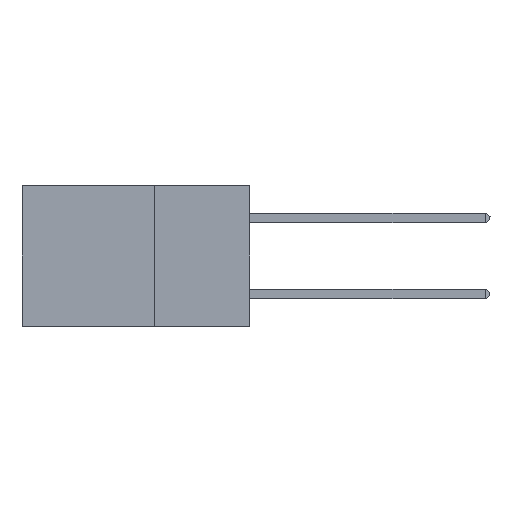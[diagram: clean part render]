
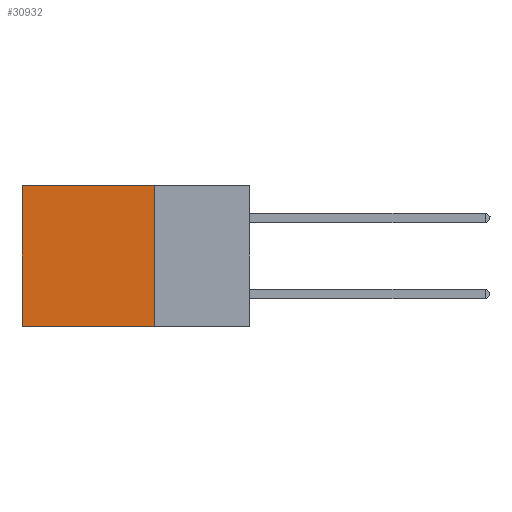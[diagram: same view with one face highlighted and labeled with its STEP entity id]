
A CAD part, left-side view. The second image highlights one B-rep face of the part: STEP entity #30932.
In plain terms, the highlighted planar face has unit normal (-1, 0, 0).
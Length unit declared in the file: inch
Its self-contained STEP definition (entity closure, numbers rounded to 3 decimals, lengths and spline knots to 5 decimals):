
#968 = VERTEX_POINT ( 'NONE', #5700 ) ;
#1613 = VERTEX_POINT ( 'NONE', #4851 ) ;
#2082 = ORIENTED_EDGE ( 'NONE', *, *, #34504, .F. ) ;
#3771 = LINE ( 'NONE', #9595, #23600 ) ;
#3951 = DIRECTION ( 'NONE',  ( 0., 0., -1. ) ) ;
#4851 = CARTESIAN_POINT ( 'NONE',  ( 0.2875, 0.6, -0.37 ) ) ;
#4903 = PLANE ( 'NONE',  #20054 ) ;
#5700 = CARTESIAN_POINT ( 'NONE',  ( 0.2875, 0.6, 0. ) ) ;
#8039 = CARTESIAN_POINT ( 'NONE',  ( 0.2875, 0.25, -0.37 ) ) ;
#9595 = CARTESIAN_POINT ( 'NONE',  ( 0.2875, 0.6, 0. ) ) ;
#10537 = FACE_OUTER_BOUND ( 'NONE', #33768, .T. ) ;
#10562 = EDGE_CURVE ( 'NONE', #968, #1613, #3771, .T. ) ;
#10902 = CARTESIAN_POINT ( 'NONE',  ( 0.2875, 0.25, 0. ) ) ;
#11236 = ORIENTED_EDGE ( 'NONE', *, *, #29408, .T. ) ;
#11435 = VECTOR ( 'NONE', #25036, 39.37008 ) ;
#13831 = DIRECTION ( 'NONE',  ( 1., 0., 0. ) ) ;
#14778 = ORIENTED_EDGE ( 'NONE', *, *, #35488, .F. ) ;
#17327 = VERTEX_POINT ( 'NONE', #25111 ) ;
#19343 = CARTESIAN_POINT ( 'NONE',  ( 0.2875, 0.25, 0. ) ) ;
#20054 = AXIS2_PLACEMENT_3D ( 'NONE', #10902, #13831, #33153 ) ;
#21034 = CARTESIAN_POINT ( 'NONE',  ( 0.2875, 0.25, -0.37 ) ) ;
#23600 = VECTOR ( 'NONE', #3951, 39.37008 ) ;
#23776 = LINE ( 'NONE', #21034, #24204 ) ;
#24204 = VECTOR ( 'NONE', #27042, 39.37008 ) ;
#24647 = VERTEX_POINT ( 'NONE', #8039 ) ;
#25036 = DIRECTION ( 'NONE',  ( 0., 0., -1. ) ) ;
#25111 = CARTESIAN_POINT ( 'NONE',  ( 0.2875, 0.25, 0. ) ) ;
#25226 = CARTESIAN_POINT ( 'NONE',  ( 0.2875, 0.25, 0. ) ) ;
#27042 = DIRECTION ( 'NONE',  ( 0., 1., 0. ) ) ;
#29408 = EDGE_CURVE ( 'NONE', #17327, #968, #35358, .T. ) ;
#30850 = LINE ( 'NONE', #25226, #11435 ) ;
#30932 = ADVANCED_FACE ( 'NONE', ( #10537 ), #4903, .F. ) ;
#31007 = VECTOR ( 'NONE', #35899, 39.37008 ) ;
#31587 = ORIENTED_EDGE ( 'NONE', *, *, #10562, .T. ) ;
#33153 = DIRECTION ( 'NONE',  ( 0., 0., -1. ) ) ;
#33768 = EDGE_LOOP ( 'NONE', ( #31587, #2082, #14778, #11236 ) ) ;
#34504 = EDGE_CURVE ( 'NONE', #24647, #1613, #23776, .T. ) ;
#35358 = LINE ( 'NONE', #19343, #31007 ) ;
#35488 = EDGE_CURVE ( 'NONE', #17327, #24647, #30850, .T. ) ;
#35899 = DIRECTION ( 'NONE',  ( 0., 1., 0. ) ) ;
